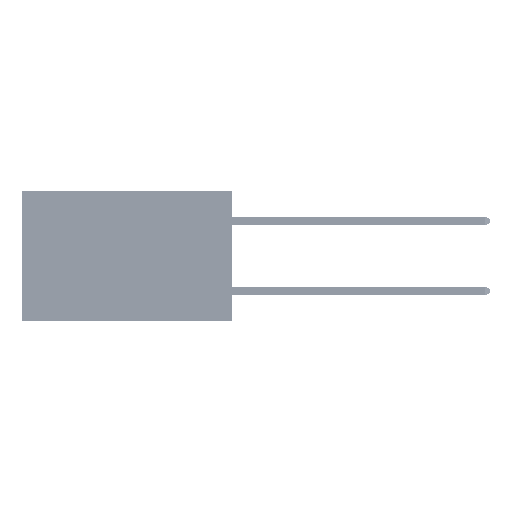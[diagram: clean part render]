
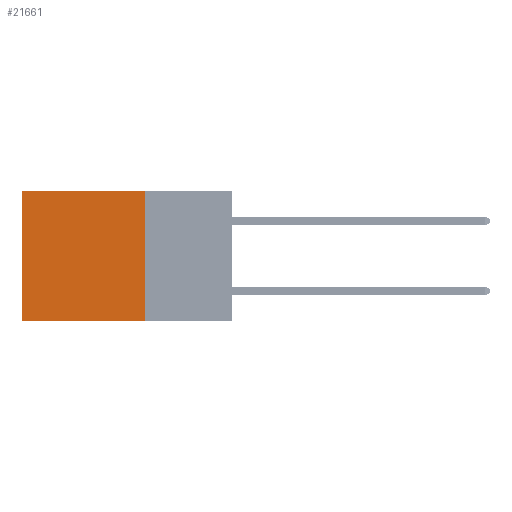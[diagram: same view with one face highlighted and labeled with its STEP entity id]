
A CAD part, left-side view. The second image highlights one B-rep face of the part: STEP entity #21661.
In plain terms, the highlighted planar face has unit normal (-1, 0, 0).
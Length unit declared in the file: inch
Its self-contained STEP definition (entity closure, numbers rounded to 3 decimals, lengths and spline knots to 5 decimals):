
#893 = CARTESIAN_POINT ( 'NONE',  ( 0.2875, 0.6, 0. ) ) ;
#1879 = LINE ( 'NONE', #37823, #5590 ) ;
#2529 = AXIS2_PLACEMENT_3D ( 'NONE', #20133, #35970, #47724 ) ;
#2565 = EDGE_CURVE ( 'NONE', #3570, #36319, #9122, .T. ) ;
#2990 = EDGE_CURVE ( 'NONE', #18372, #3570, #12131, .T. ) ;
#3570 = VERTEX_POINT ( 'NONE', #18196 ) ;
#5590 = VECTOR ( 'NONE', #13878, 39.37008 ) ;
#7896 = CARTESIAN_POINT ( 'NONE',  ( 0.2875, 0.25, -0.37 ) ) ;
#8429 = PLANE ( 'NONE',  #2529 ) ;
#9122 = LINE ( 'NONE', #893, #20821 ) ;
#10954 = EDGE_LOOP ( 'NONE', ( #19460, #17587, #18554, #12349 ) ) ;
#12055 = CARTESIAN_POINT ( 'NONE',  ( 0.2875, 0.25, -0.37 ) ) ;
#12131 = LINE ( 'NONE', #42868, #35550 ) ;
#12349 = ORIENTED_EDGE ( 'NONE', *, *, #2990, .T. ) ;
#13878 = DIRECTION ( 'NONE',  ( 0., 0., -1. ) ) ;
#14568 = EDGE_CURVE ( 'NONE', #18372, #36887, #1879, .T. ) ;
#15123 = DIRECTION ( 'NONE',  ( 0., 1., 0. ) ) ;
#16216 = DIRECTION ( 'NONE',  ( 0., 0., -1. ) ) ;
#17587 = ORIENTED_EDGE ( 'NONE', *, *, #37537, .F. ) ;
#18196 = CARTESIAN_POINT ( 'NONE',  ( 0.2875, 0.6, 0. ) ) ;
#18372 = VERTEX_POINT ( 'NONE', #39619 ) ;
#18554 = ORIENTED_EDGE ( 'NONE', *, *, #14568, .F. ) ;
#19460 = ORIENTED_EDGE ( 'NONE', *, *, #2565, .T. ) ;
#20133 = CARTESIAN_POINT ( 'NONE',  ( 0.2875, 0.25, 0. ) ) ;
#20175 = LINE ( 'NONE', #7896, #33687 ) ;
#20821 = VECTOR ( 'NONE', #16216, 39.37008 ) ;
#21661 = ADVANCED_FACE ( 'NONE', ( #31020 ), #8429, .F. ) ;
#22158 = CARTESIAN_POINT ( 'NONE',  ( 0.2875, 0.6, -0.37 ) ) ;
#31020 = FACE_OUTER_BOUND ( 'NONE', #10954, .T. ) ;
#33687 = VECTOR ( 'NONE', #15123, 39.37008 ) ;
#35550 = VECTOR ( 'NONE', #50453, 39.37008 ) ;
#35970 = DIRECTION ( 'NONE',  ( 1., 0., 0. ) ) ;
#36319 = VERTEX_POINT ( 'NONE', #22158 ) ;
#36887 = VERTEX_POINT ( 'NONE', #12055 ) ;
#37537 = EDGE_CURVE ( 'NONE', #36887, #36319, #20175, .T. ) ;
#37823 = CARTESIAN_POINT ( 'NONE',  ( 0.2875, 0.25, 0. ) ) ;
#39619 = CARTESIAN_POINT ( 'NONE',  ( 0.2875, 0.25, 0. ) ) ;
#42868 = CARTESIAN_POINT ( 'NONE',  ( 0.2875, 0.25, 0. ) ) ;
#47724 = DIRECTION ( 'NONE',  ( 0., 0., -1. ) ) ;
#50453 = DIRECTION ( 'NONE',  ( 0., 1., 0. ) ) ;
